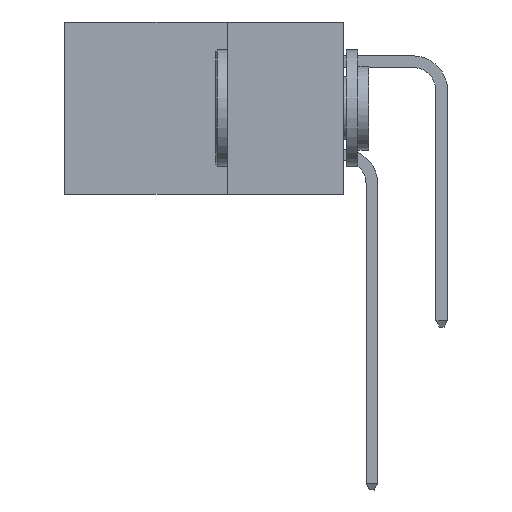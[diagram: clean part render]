
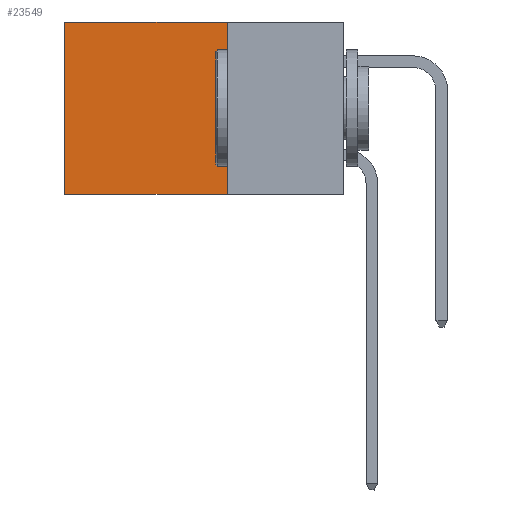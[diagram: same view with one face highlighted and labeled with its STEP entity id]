
A CAD part, left-side view. The second image highlights one B-rep face of the part: STEP entity #23549.
In plain terms, the highlighted planar face has unit normal (-1, 0, 0).
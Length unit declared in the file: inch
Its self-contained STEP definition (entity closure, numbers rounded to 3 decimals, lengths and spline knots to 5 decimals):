
#827 = DIRECTION ( 'NONE',  ( 0., 0., -1. ) ) ;
#1042 = ORIENTED_EDGE ( 'NONE', *, *, #25416, .F. ) ;
#1742 = VECTOR ( 'NONE', #1832, 39.37008 ) ;
#1832 = DIRECTION ( 'NONE',  ( 0., 1., 0. ) ) ;
#2644 = EDGE_CURVE ( 'NONE', #16753, #4402, #25677, .T. ) ;
#3088 = VECTOR ( 'NONE', #16944, 39.37008 ) ;
#3866 = CARTESIAN_POINT ( 'NONE',  ( 0.2615, 0.25, 0. ) ) ;
#3912 = LINE ( 'NONE', #18475, #1742 ) ;
#4082 = EDGE_CURVE ( 'NONE', #10618, #24833, #3912, .T. ) ;
#4402 = VERTEX_POINT ( 'NONE', #26391 ) ;
#5093 = DIRECTION ( 'NONE',  ( 0., 1., 0. ) ) ;
#6254 = CARTESIAN_POINT ( 'NONE',  ( 0.2615, 0.25, -0.37 ) ) ;
#7103 = EDGE_LOOP ( 'NONE', ( #14277, #26353, #1042, #12132 ) ) ;
#7132 = CARTESIAN_POINT ( 'NONE',  ( 0.2615, 0.25, -0.37 ) ) ;
#7313 = CARTESIAN_POINT ( 'NONE',  ( 0.2615, 0.25, 0. ) ) ;
#7946 = AXIS2_PLACEMENT_3D ( 'NONE', #7132, #21818, #8776 ) ;
#8403 = CARTESIAN_POINT ( 'NONE',  ( 0.2615, 0.6, -0.37 ) ) ;
#8776 = DIRECTION ( 'NONE',  ( 0., 0., -1. ) ) ;
#10515 = LINE ( 'NONE', #6254, #3088 ) ;
#10618 = VERTEX_POINT ( 'NONE', #21030 ) ;
#10863 = PLANE ( 'NONE',  #7946 ) ;
#12132 = ORIENTED_EDGE ( 'NONE', *, *, #2644, .T. ) ;
#14045 = EDGE_CURVE ( 'NONE', #4402, #24833, #15816, .T. ) ;
#14277 = ORIENTED_EDGE ( 'NONE', *, *, #14045, .T. ) ;
#15816 = LINE ( 'NONE', #17761, #24277 ) ;
#16753 = VERTEX_POINT ( 'NONE', #3866 ) ;
#16944 = DIRECTION ( 'NONE',  ( 0., 0., -1. ) ) ;
#17761 = CARTESIAN_POINT ( 'NONE',  ( 0.2615, 0.6, -0.37 ) ) ;
#18475 = CARTESIAN_POINT ( 'NONE',  ( 0.2615, 0.25, -0.37 ) ) ;
#21030 = CARTESIAN_POINT ( 'NONE',  ( 0.2615, 0.25, -0.37 ) ) ;
#21818 = DIRECTION ( 'NONE',  ( 1., 0., 0. ) ) ;
#22077 = VECTOR ( 'NONE', #5093, 39.37008 ) ;
#23549 = ADVANCED_FACE ( 'NONE', ( #23799 ), #10863, .F. ) ;
#23799 = FACE_OUTER_BOUND ( 'NONE', #7103, .T. ) ;
#24277 = VECTOR ( 'NONE', #827, 39.37008 ) ;
#24833 = VERTEX_POINT ( 'NONE', #8403 ) ;
#25416 = EDGE_CURVE ( 'NONE', #16753, #10618, #10515, .T. ) ;
#25677 = LINE ( 'NONE', #7313, #22077 ) ;
#26353 = ORIENTED_EDGE ( 'NONE', *, *, #4082, .F. ) ;
#26391 = CARTESIAN_POINT ( 'NONE',  ( 0.2615, 0.6, 0. ) ) ;
